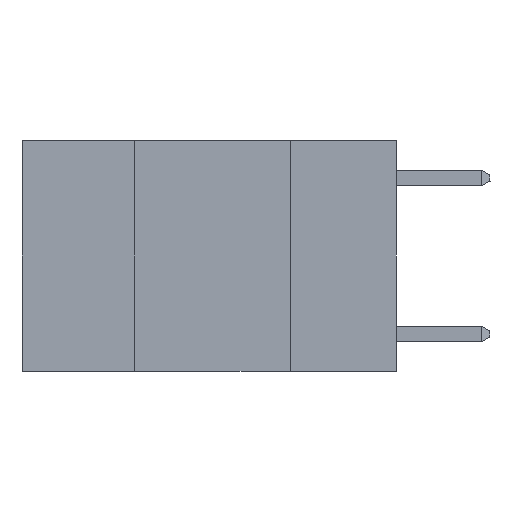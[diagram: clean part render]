
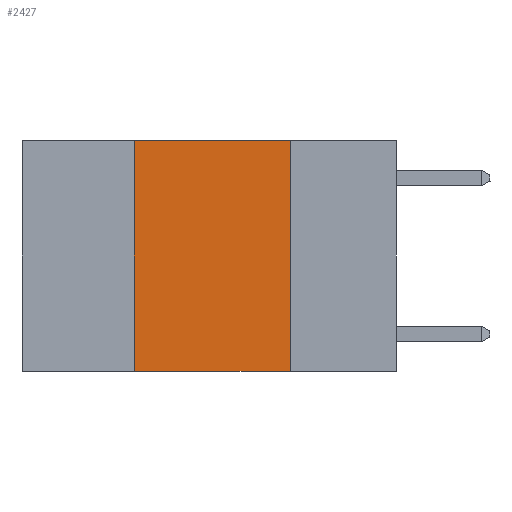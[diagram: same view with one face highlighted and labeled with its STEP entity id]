
A CAD part, left-side view. The second image highlights one B-rep face of the part: STEP entity #2427.
In plain terms, the highlighted planar face has unit normal (-1, 0, 0).
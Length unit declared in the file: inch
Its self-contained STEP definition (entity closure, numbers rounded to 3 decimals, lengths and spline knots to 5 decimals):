
#210 = CARTESIAN_POINT ( 'NONE',  ( 0., 0.6, 0. ) ) ;
#981 = EDGE_CURVE ( 'NONE', #14959, #4721, #10253, .T. ) ;
#1336 = ORIENTED_EDGE ( 'NONE', *, *, #981, .T. ) ;
#1377 = CARTESIAN_POINT ( 'NONE',  ( 0., 0.6, 0. ) ) ;
#1519 = DIRECTION ( 'NONE',  ( 1., 0., 0. ) ) ;
#1601 = CARTESIAN_POINT ( 'NONE',  ( 0., 0.42, 0. ) ) ;
#2120 = CARTESIAN_POINT ( 'NONE',  ( 0., 0.42, 0. ) ) ;
#2427 = ADVANCED_FACE ( 'NONE', ( #5100 ), #8028, .F. ) ;
#3851 = CARTESIAN_POINT ( 'NONE',  ( 0., 0.17, -0.37 ) ) ;
#4289 = VECTOR ( 'NONE', #5511, 39.37008 ) ;
#4584 = ORIENTED_EDGE ( 'NONE', *, *, #10039, .F. ) ;
#4721 = VERTEX_POINT ( 'NONE', #3851 ) ;
#5100 = FACE_OUTER_BOUND ( 'NONE', #10718, .T. ) ;
#5511 = DIRECTION ( 'NONE',  ( 0., 0., 1. ) ) ;
#5514 = EDGE_CURVE ( 'NONE', #13431, #9971, #15996, .T. ) ;
#6021 = VECTOR ( 'NONE', #10506, 39.37008 ) ;
#7237 = DIRECTION ( 'NONE',  ( 0., -1., 0. ) ) ;
#7768 = LINE ( 'NONE', #1601, #4289 ) ;
#8028 = PLANE ( 'NONE',  #11447 ) ;
#8237 = LINE ( 'NONE', #16386, #13901 ) ;
#9126 = CARTESIAN_POINT ( 'NONE',  ( 0., 0.6, -0.37 ) ) ;
#9971 = VERTEX_POINT ( 'NONE', #13697 ) ;
#10039 = EDGE_CURVE ( 'NONE', #9971, #4721, #8237, .T. ) ;
#10253 = LINE ( 'NONE', #9126, #13293 ) ;
#10506 = DIRECTION ( 'NONE',  ( 0., -1., 0. ) ) ;
#10638 = DIRECTION ( 'NONE',  ( 0., 0., -1. ) ) ;
#10718 = EDGE_LOOP ( 'NONE', ( #4584, #16595, #13939, #1336 ) ) ;
#11447 = AXIS2_PLACEMENT_3D ( 'NONE', #210, #1519, #10638 ) ;
#11788 = EDGE_CURVE ( 'NONE', #14959, #13431, #7768, .T. ) ;
#12967 = CARTESIAN_POINT ( 'NONE',  ( 0., 0.42, -0.37 ) ) ;
#13293 = VECTOR ( 'NONE', #7237, 39.37008 ) ;
#13431 = VERTEX_POINT ( 'NONE', #2120 ) ;
#13697 = CARTESIAN_POINT ( 'NONE',  ( 0., 0.17, 0. ) ) ;
#13901 = VECTOR ( 'NONE', #16318, 39.37008 ) ;
#13939 = ORIENTED_EDGE ( 'NONE', *, *, #11788, .F. ) ;
#14959 = VERTEX_POINT ( 'NONE', #12967 ) ;
#15996 = LINE ( 'NONE', #1377, #6021 ) ;
#16318 = DIRECTION ( 'NONE',  ( 0., 0., -1. ) ) ;
#16386 = CARTESIAN_POINT ( 'NONE',  ( 0., 0.17, 0. ) ) ;
#16595 = ORIENTED_EDGE ( 'NONE', *, *, #5514, .F. ) ;
